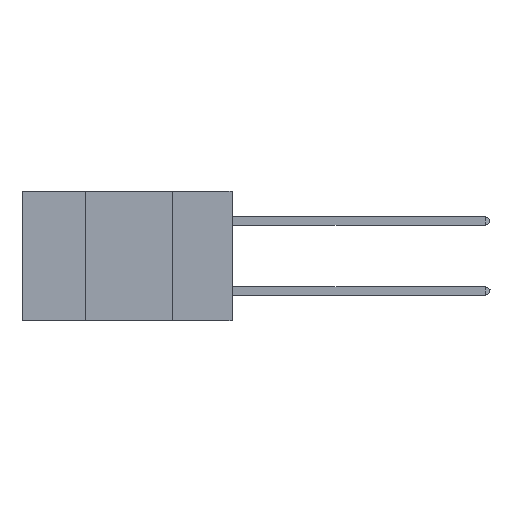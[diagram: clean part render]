
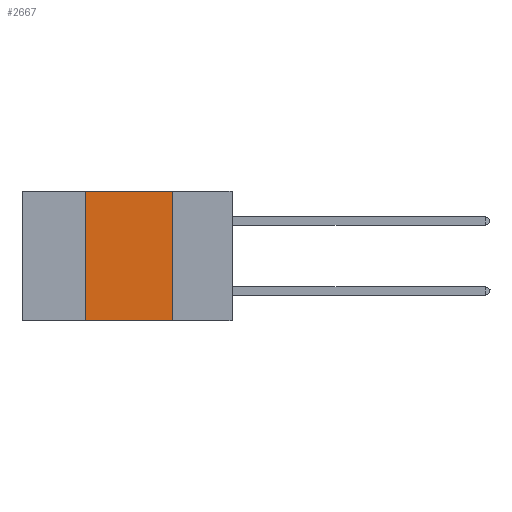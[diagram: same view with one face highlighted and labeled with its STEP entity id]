
A CAD part, left-side view. The second image highlights one B-rep face of the part: STEP entity #2667.
In plain terms, the highlighted planar face has unit normal (-1, 0, 0).
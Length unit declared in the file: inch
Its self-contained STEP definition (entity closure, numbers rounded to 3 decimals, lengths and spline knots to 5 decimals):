
#570 = CARTESIAN_POINT ( 'NONE',  ( 0., 0.6, -0.37 ) ) ;
#1103 = EDGE_CURVE ( 'NONE', #2795, #3059, #2203, .T. ) ;
#1434 = DIRECTION ( 'NONE',  ( 0., -1., 0. ) ) ;
#2203 = LINE ( 'NONE', #570, #12822 ) ;
#2667 = ADVANCED_FACE ( 'NONE', ( #4604 ), #16216, .F. ) ;
#2795 = VERTEX_POINT ( 'NONE', #15465 ) ;
#3059 = VERTEX_POINT ( 'NONE', #14720 ) ;
#3292 = DIRECTION ( 'NONE',  ( 0., 0., 1. ) ) ;
#4027 = EDGE_CURVE ( 'NONE', #5309, #7210, #14181, .T. ) ;
#4041 = CARTESIAN_POINT ( 'NONE',  ( 0., 0.6, 0. ) ) ;
#4408 = VECTOR ( 'NONE', #1434, 39.37008 ) ;
#4604 = FACE_OUTER_BOUND ( 'NONE', #10204, .T. ) ;
#5309 = VERTEX_POINT ( 'NONE', #11073 ) ;
#5387 = DIRECTION ( 'NONE',  ( 0., 0., -1. ) ) ;
#7154 = ORIENTED_EDGE ( 'NONE', *, *, #4027, .F. ) ;
#7210 = VERTEX_POINT ( 'NONE', #13331 ) ;
#8126 = ORIENTED_EDGE ( 'NONE', *, *, #15879, .F. ) ;
#8780 = LINE ( 'NONE', #14397, #15061 ) ;
#9257 = DIRECTION ( 'NONE',  ( 0., 0., -1. ) ) ;
#10204 = EDGE_LOOP ( 'NONE', ( #8126, #7154, #14513, #16342 ) ) ;
#11073 = CARTESIAN_POINT ( 'NONE',  ( 0., 0.42, 0. ) ) ;
#12254 = CARTESIAN_POINT ( 'NONE',  ( 0., 0.6, 0. ) ) ;
#12705 = EDGE_CURVE ( 'NONE', #2795, #5309, #8780, .T. ) ;
#12822 = VECTOR ( 'NONE', #13089, 39.37008 ) ;
#13089 = DIRECTION ( 'NONE',  ( 0., -1., 0. ) ) ;
#13331 = CARTESIAN_POINT ( 'NONE',  ( 0., 0.17, 0. ) ) ;
#14156 = LINE ( 'NONE', #14738, #14571 ) ;
#14181 = LINE ( 'NONE', #4041, #4408 ) ;
#14347 = AXIS2_PLACEMENT_3D ( 'NONE', #12254, #16459, #9257 ) ;
#14397 = CARTESIAN_POINT ( 'NONE',  ( 0., 0.42, 0. ) ) ;
#14513 = ORIENTED_EDGE ( 'NONE', *, *, #12705, .F. ) ;
#14571 = VECTOR ( 'NONE', #5387, 39.37008 ) ;
#14720 = CARTESIAN_POINT ( 'NONE',  ( 0., 0.17, -0.37 ) ) ;
#14738 = CARTESIAN_POINT ( 'NONE',  ( 0., 0.17, 0. ) ) ;
#15061 = VECTOR ( 'NONE', #3292, 39.37008 ) ;
#15465 = CARTESIAN_POINT ( 'NONE',  ( 0., 0.42, -0.37 ) ) ;
#15879 = EDGE_CURVE ( 'NONE', #7210, #3059, #14156, .T. ) ;
#16216 = PLANE ( 'NONE',  #14347 ) ;
#16342 = ORIENTED_EDGE ( 'NONE', *, *, #1103, .T. ) ;
#16459 = DIRECTION ( 'NONE',  ( 1., 0., 0. ) ) ;
